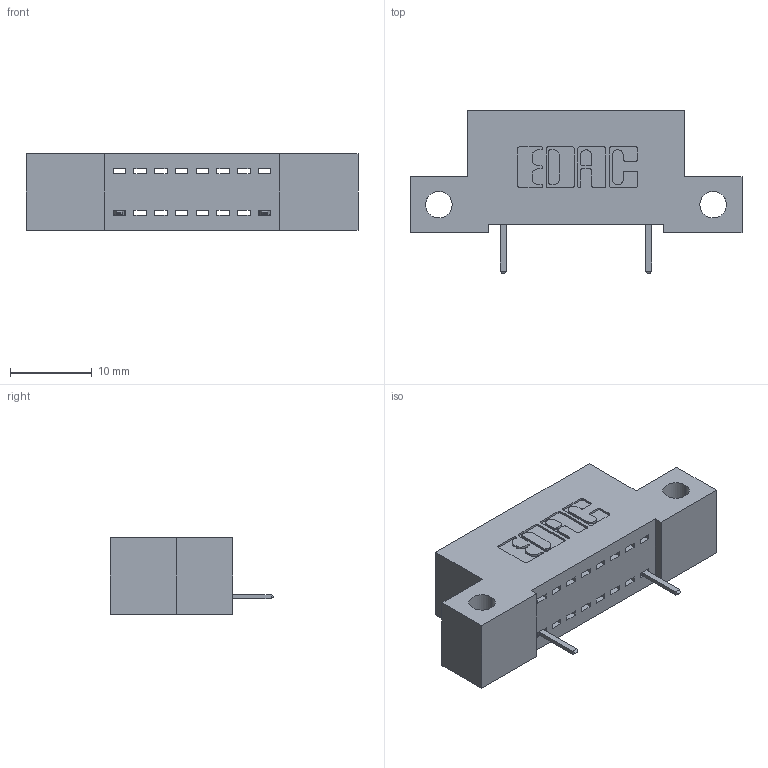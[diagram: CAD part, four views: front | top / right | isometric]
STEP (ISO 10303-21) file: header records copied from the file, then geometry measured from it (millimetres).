
FILE_DESCRIPTION (( 'STEP AP203' ), '1' );
FILE_NAME ('392-008-520-112.STEP', '2018-08-14T19:08:52', ( '' ), ( '' ), 'SwSTEP 2.0', 'SolidWorks 2016', '' );
FILE_SCHEMA (( 'CONFIG_CONTROL_DESIGN' ));
Length unit declared in the file: inch
Products named in the file (3): 342 Part_Side Mount; 345-292-001_345-293-120; 392-008-520-112
Assembly tree (3 placements, depth 2):
  392-008-520-112
    342 Part_Side Mount
    345-292-001_345-293-120  x2
Bounding box: 40.64 x 20.02 x 9.4 mm (x, y, z)
Volume: 3289.8 mm3; surface area: 3659 mm2
Topology: 3 solids, 3 shells, 306 faces, 919 edges, 606 vertices
Faces by surface type: plane 226, cylinder 80
Entity records: 9081 total; most frequent: CARTESIAN_POINT 1616, ORIENTED_EDGE 1554, DIRECTION 1413, EDGE_CURVE 777, LINE 645, VECTOR 645, VERTEX_POINT 514, AXIS2_PLACEMENT_3D 384
